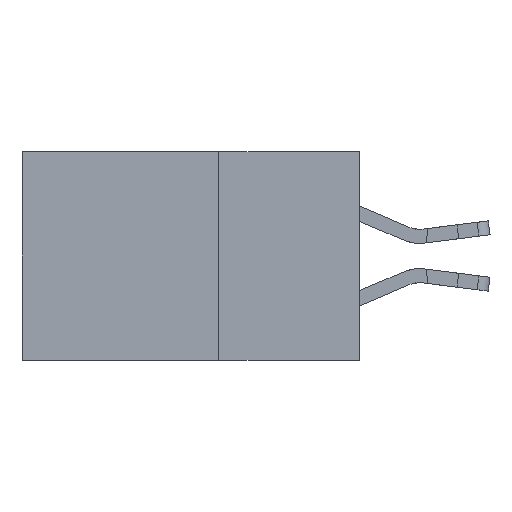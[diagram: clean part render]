
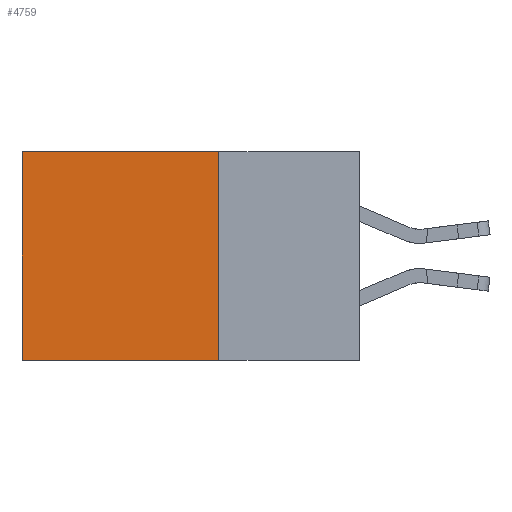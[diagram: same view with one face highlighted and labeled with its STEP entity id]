
A CAD part, left-side view. The second image highlights one B-rep face of the part: STEP entity #4759.
In plain terms, the highlighted planar face has unit normal (-1, 0, 0).
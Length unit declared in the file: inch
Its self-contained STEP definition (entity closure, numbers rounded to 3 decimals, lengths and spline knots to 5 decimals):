
#236 = ORIENTED_EDGE ( 'NONE', *, *, #6252, .F. ) ;
#933 = EDGE_CURVE ( 'NONE', #7389, #1695, #13864, .T. ) ;
#1593 = LINE ( 'NONE', #16879, #22531 ) ;
#1695 = VERTEX_POINT ( 'NONE', #3771 ) ;
#2011 = DIRECTION ( 'NONE',  ( 1., 0., 0. ) ) ;
#2105 = CARTESIAN_POINT ( 'NONE',  ( 0.2875, 0.25, -0.37 ) ) ;
#2117 = ORIENTED_EDGE ( 'NONE', *, *, #933, .T. ) ;
#2450 = ORIENTED_EDGE ( 'NONE', *, *, #7384, .T. ) ;
#3447 = LINE ( 'NONE', #2105, #21043 ) ;
#3552 = CARTESIAN_POINT ( 'NONE',  ( 0.2875, 0.25, -0.37 ) ) ;
#3609 = EDGE_LOOP ( 'NONE', ( #2450, #236, #22172, #2117 ) ) ;
#3771 = CARTESIAN_POINT ( 'NONE',  ( 0.2875, 0.6, 0. ) ) ;
#4206 = VERTEX_POINT ( 'NONE', #3552 ) ;
#4759 = ADVANCED_FACE ( 'NONE', ( #5736 ), #6562, .F. ) ;
#4927 = AXIS2_PLACEMENT_3D ( 'NONE', #12613, #2011, #7326 ) ;
#5736 = FACE_OUTER_BOUND ( 'NONE', #3609, .T. ) ;
#6252 = EDGE_CURVE ( 'NONE', #4206, #15847, #3447, .T. ) ;
#6562 = PLANE ( 'NONE',  #4927 ) ;
#7326 = DIRECTION ( 'NONE',  ( 0., 0., -1. ) ) ;
#7384 = EDGE_CURVE ( 'NONE', #1695, #15847, #18650, .T. ) ;
#7389 = VERTEX_POINT ( 'NONE', #12409 ) ;
#8522 = CARTESIAN_POINT ( 'NONE',  ( 0.2875, 0.6, 0. ) ) ;
#8602 = DIRECTION ( 'NONE',  ( 0., 0., -1. ) ) ;
#9442 = VECTOR ( 'NONE', #15721, 39.37008 ) ;
#11562 = EDGE_CURVE ( 'NONE', #7389, #4206, #1593, .T. ) ;
#12065 = VECTOR ( 'NONE', #8602, 39.37008 ) ;
#12409 = CARTESIAN_POINT ( 'NONE',  ( 0.2875, 0.25, 0. ) ) ;
#12613 = CARTESIAN_POINT ( 'NONE',  ( 0.2875, 0.25, 0. ) ) ;
#13864 = LINE ( 'NONE', #17688, #9442 ) ;
#15721 = DIRECTION ( 'NONE',  ( 0., 1., 0. ) ) ;
#15847 = VERTEX_POINT ( 'NONE', #19370 ) ;
#16879 = CARTESIAN_POINT ( 'NONE',  ( 0.2875, 0.25, 0. ) ) ;
#16952 = DIRECTION ( 'NONE',  ( 0., 0., -1. ) ) ;
#17688 = CARTESIAN_POINT ( 'NONE',  ( 0.2875, 0.25, 0. ) ) ;
#18650 = LINE ( 'NONE', #8522, #12065 ) ;
#19370 = CARTESIAN_POINT ( 'NONE',  ( 0.2875, 0.6, -0.37 ) ) ;
#21043 = VECTOR ( 'NONE', #21192, 39.37008 ) ;
#21192 = DIRECTION ( 'NONE',  ( 0., 1., 0. ) ) ;
#22172 = ORIENTED_EDGE ( 'NONE', *, *, #11562, .F. ) ;
#22531 = VECTOR ( 'NONE', #16952, 39.37008 ) ;
